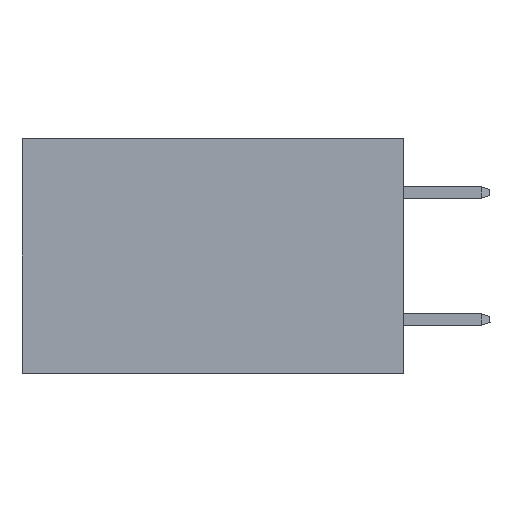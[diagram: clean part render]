
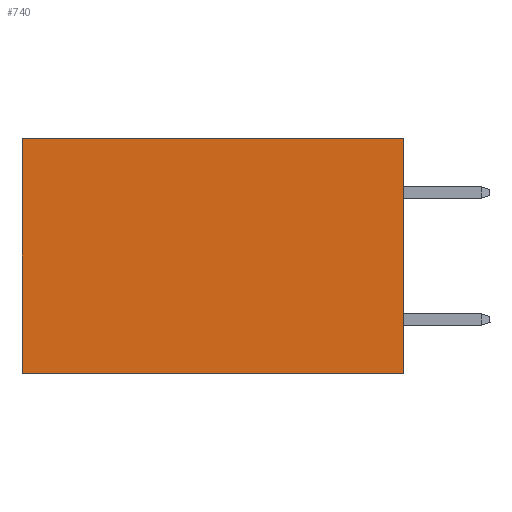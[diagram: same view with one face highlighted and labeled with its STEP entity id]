
A CAD part, left-side view. The second image highlights one B-rep face of the part: STEP entity #740.
In plain terms, the highlighted planar face has unit normal (-1, 0, 0).
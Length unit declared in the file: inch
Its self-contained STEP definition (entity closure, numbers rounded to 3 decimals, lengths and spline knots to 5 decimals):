
#123 = EDGE_CURVE ( 'NONE', #9441, #6791, #1517, .T. ) ;
#255 = CARTESIAN_POINT ( 'NONE',  ( 0.2875, 0., 0. ) ) ;
#563 = DIRECTION ( 'NONE',  ( 0., 0., -1. ) ) ;
#620 = DIRECTION ( 'NONE',  ( 0., 0., -1. ) ) ;
#740 = ADVANCED_FACE ( 'NONE', ( #3308 ), #13763, .F. ) ;
#1203 = EDGE_CURVE ( 'NONE', #15584, #6099, #15139, .T. ) ;
#1281 = DIRECTION ( 'NONE',  ( 0., 0., -1. ) ) ;
#1327 = VECTOR ( 'NONE', #3179, 39.37008 ) ;
#1342 = EDGE_LOOP ( 'NONE', ( #6276, #2953, #9664, #10261 ) ) ;
#1517 = LINE ( 'NONE', #255, #2235 ) ;
#1995 = CARTESIAN_POINT ( 'NONE',  ( 0.2875, 0., 0. ) ) ;
#2235 = VECTOR ( 'NONE', #563, 39.37008 ) ;
#2617 = CARTESIAN_POINT ( 'NONE',  ( 0.2875, 0.6, -0.37 ) ) ;
#2953 = ORIENTED_EDGE ( 'NONE', *, *, #14226, .F. ) ;
#3179 = DIRECTION ( 'NONE',  ( 0., 1., 0. ) ) ;
#3232 = EDGE_CURVE ( 'NONE', #9441, #15584, #16031, .T. ) ;
#3308 = FACE_OUTER_BOUND ( 'NONE', #1342, .T. ) ;
#3760 = VECTOR ( 'NONE', #12469, 39.37008 ) ;
#4494 = CARTESIAN_POINT ( 'NONE',  ( 0.2875, 0., 0. ) ) ;
#6099 = VERTEX_POINT ( 'NONE', #2617 ) ;
#6276 = ORIENTED_EDGE ( 'NONE', *, *, #1203, .T. ) ;
#6791 = VERTEX_POINT ( 'NONE', #12094 ) ;
#7067 = AXIS2_PLACEMENT_3D ( 'NONE', #7325, #7412, #620 ) ;
#7325 = CARTESIAN_POINT ( 'NONE',  ( 0.2875, 0., 0. ) ) ;
#7412 = DIRECTION ( 'NONE',  ( 1., 0., 0. ) ) ;
#7631 = VECTOR ( 'NONE', #1281, 39.37008 ) ;
#9441 = VERTEX_POINT ( 'NONE', #4494 ) ;
#9664 = ORIENTED_EDGE ( 'NONE', *, *, #123, .F. ) ;
#10133 = LINE ( 'NONE', #15220, #3760 ) ;
#10261 = ORIENTED_EDGE ( 'NONE', *, *, #3232, .T. ) ;
#10704 = CARTESIAN_POINT ( 'NONE',  ( 0.2875, 0.6, 0. ) ) ;
#12094 = CARTESIAN_POINT ( 'NONE',  ( 0.2875, 0., -0.37 ) ) ;
#12469 = DIRECTION ( 'NONE',  ( 0., 1., 0. ) ) ;
#13763 = PLANE ( 'NONE',  #7067 ) ;
#13821 = CARTESIAN_POINT ( 'NONE',  ( 0.2875, 0.6, 0. ) ) ;
#14226 = EDGE_CURVE ( 'NONE', #6791, #6099, #10133, .T. ) ;
#15139 = LINE ( 'NONE', #13821, #7631 ) ;
#15220 = CARTESIAN_POINT ( 'NONE',  ( 0.2875, 0., -0.37 ) ) ;
#15584 = VERTEX_POINT ( 'NONE', #10704 ) ;
#16031 = LINE ( 'NONE', #1995, #1327 ) ;
